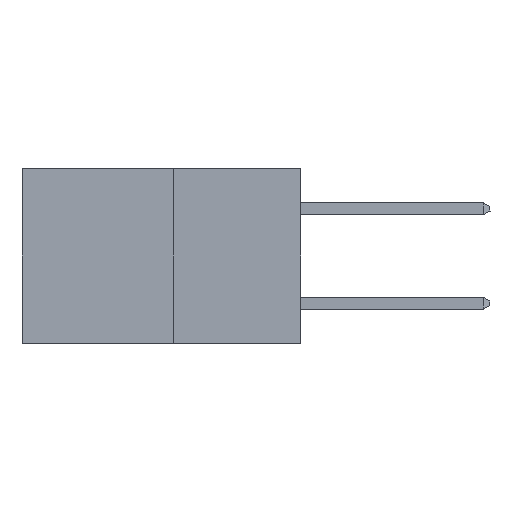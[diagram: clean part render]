
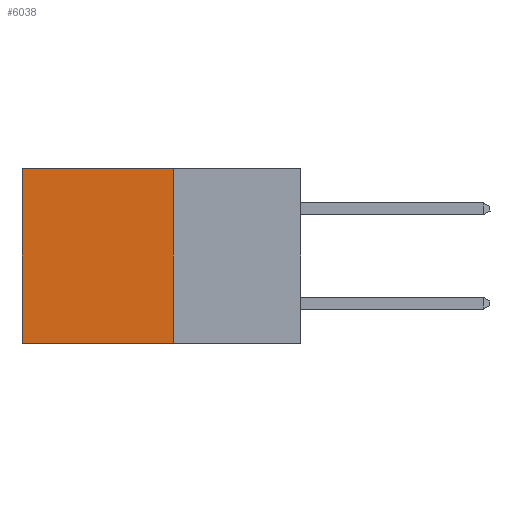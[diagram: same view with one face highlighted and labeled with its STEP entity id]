
A CAD part, left-side view. The second image highlights one B-rep face of the part: STEP entity #6038.
In plain terms, the highlighted planar face has unit normal (-1, 0, 0).
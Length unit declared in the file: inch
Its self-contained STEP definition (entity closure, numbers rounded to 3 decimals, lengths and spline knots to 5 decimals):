
#7 = CARTESIAN_POINT ( 'NONE',  ( 0.277, 0.27, -0.37 ) ) ;
#322 = VECTOR ( 'NONE', #15666, 39.37008 ) ;
#1359 = CARTESIAN_POINT ( 'NONE',  ( 0.277, 0.27, -0.37 ) ) ;
#3386 = PLANE ( 'NONE',  #5649 ) ;
#4567 = LINE ( 'NONE', #7, #322 ) ;
#4943 = DIRECTION ( 'NONE',  ( 0., 0., -1. ) ) ;
#4972 = DIRECTION ( 'NONE',  ( 1., 0., 0. ) ) ;
#5255 = DIRECTION ( 'NONE',  ( 0., 0., -1. ) ) ;
#5649 = AXIS2_PLACEMENT_3D ( 'NONE', #19027, #4972, #4943 ) ;
#6038 = ADVANCED_FACE ( 'NONE', ( #13998 ), #3386, .F. ) ;
#6210 = EDGE_LOOP ( 'NONE', ( #12054, #16406, #13459, #16873 ) ) ;
#6606 = EDGE_CURVE ( 'NONE', #19106, #13472, #15554, .T. ) ;
#6666 = CARTESIAN_POINT ( 'NONE',  ( 0.277, 0.27, 0. ) ) ;
#6931 = VECTOR ( 'NONE', #5255, 39.37008 ) ;
#8152 = DIRECTION ( 'NONE',  ( 0., 1., 0. ) ) ;
#8158 = CARTESIAN_POINT ( 'NONE',  ( 0.277, 0.59, -0.37 ) ) ;
#8191 = CARTESIAN_POINT ( 'NONE',  ( 0.277, 0.27, -0.37 ) ) ;
#8245 = EDGE_CURVE ( 'NONE', #8689, #13472, #18688, .T. ) ;
#8689 = VERTEX_POINT ( 'NONE', #1359 ) ;
#8739 = EDGE_CURVE ( 'NONE', #18107, #8689, #4567, .T. ) ;
#8850 = EDGE_CURVE ( 'NONE', #18107, #19106, #13961, .T. ) ;
#10954 = VECTOR ( 'NONE', #8152, 39.37008 ) ;
#11559 = DIRECTION ( 'NONE',  ( 0., 1., 0. ) ) ;
#12054 = ORIENTED_EDGE ( 'NONE', *, *, #6606, .T. ) ;
#13459 = ORIENTED_EDGE ( 'NONE', *, *, #8739, .F. ) ;
#13472 = VERTEX_POINT ( 'NONE', #8158 ) ;
#13508 = VECTOR ( 'NONE', #11559, 39.37008 ) ;
#13961 = LINE ( 'NONE', #14481, #13508 ) ;
#13998 = FACE_OUTER_BOUND ( 'NONE', #6210, .T. ) ;
#14481 = CARTESIAN_POINT ( 'NONE',  ( 0.277, 0.27, 0. ) ) ;
#15554 = LINE ( 'NONE', #16617, #6931 ) ;
#15666 = DIRECTION ( 'NONE',  ( 0., 0., -1. ) ) ;
#16406 = ORIENTED_EDGE ( 'NONE', *, *, #8245, .F. ) ;
#16617 = CARTESIAN_POINT ( 'NONE',  ( 0.277, 0.59, -0.37 ) ) ;
#16873 = ORIENTED_EDGE ( 'NONE', *, *, #8850, .T. ) ;
#16920 = CARTESIAN_POINT ( 'NONE',  ( 0.277, 0.59, 0. ) ) ;
#18107 = VERTEX_POINT ( 'NONE', #6666 ) ;
#18688 = LINE ( 'NONE', #8191, #10954 ) ;
#19027 = CARTESIAN_POINT ( 'NONE',  ( 0.277, 0.27, -0.37 ) ) ;
#19106 = VERTEX_POINT ( 'NONE', #16920 ) ;
